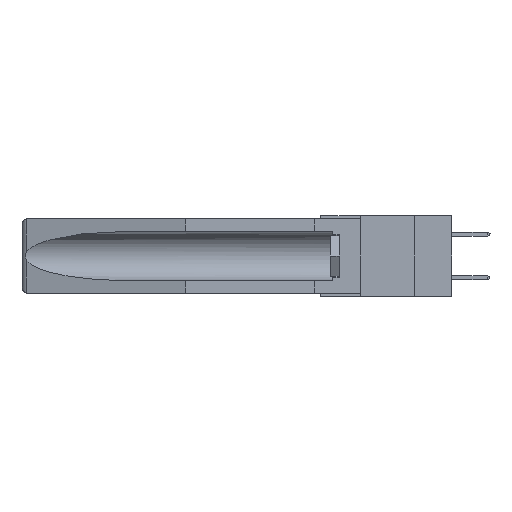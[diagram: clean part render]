
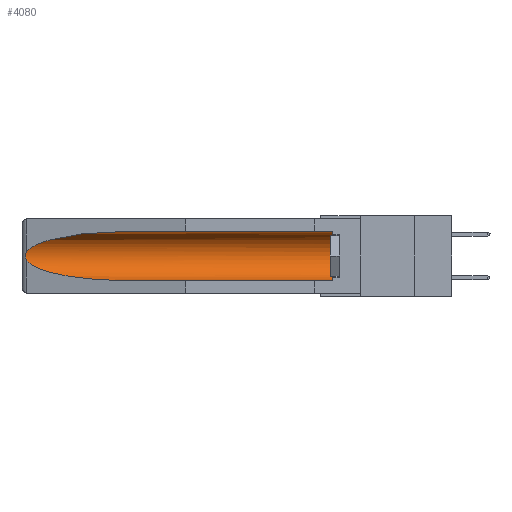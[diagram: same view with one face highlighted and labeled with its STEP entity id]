
A CAD part, left-side view. The second image highlights one B-rep face of the part: STEP entity #4080.
In plain terms, the highlighted cylindrical face has radius 2.857 mm (diameter 5.715 mm), a partial arc.
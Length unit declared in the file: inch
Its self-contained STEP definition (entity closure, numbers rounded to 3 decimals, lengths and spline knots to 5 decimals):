
#59 = LINE ( 'NONE', #6340, #12403 ) ;
#96 = ORIENTED_EDGE ( 'NONE', *, *, #6446, .F. ) ;
#229 = EDGE_CURVE ( 'NONE', #886, #3512, #5352, .T. ) ;
#364 = CARTESIAN_POINT ( 'NONE',  ( 0.26537, 1.52718, -0.14972 ) ) ;
#886 = VERTEX_POINT ( 'NONE', #3057 ) ;
#1136 = EDGE_CURVE ( 'NONE', #8082, #19232, #3600, .T. ) ;
#1971 = EDGE_CURVE ( 'NONE', #3512, #8082, #18504, .T. ) ;
#1979 = CYLINDRICAL_SURFACE ( 'NONE', #12974, 0.1125 ) ;
#2061 = CARTESIAN_POINT ( 'NONE',  ( 0.26655, 1.53094, -0.18657 ) ) ;
#2127 = CARTESIAN_POINT ( 'NONE',  ( 0.26597, 1.5296, -0.19026 ) ) ;
#3057 = CARTESIAN_POINT ( 'NONE',  ( 0.155, 1.07973, -0.059 ) ) ;
#3501 = VERTEX_POINT ( 'NONE', #14942 ) ;
#3512 = VERTEX_POINT ( 'NONE', #10009 ) ;
#3600 =( BOUNDED_CURVE ( )  B_SPLINE_CURVE ( 3, ( #16411, #5710, #16742, #4212 ),
 .UNSPECIFIED., .F., .F. ) 
 B_SPLINE_CURVE_WITH_KNOTS ( ( 4, 4 ),
 ( 0.1948, 1.5708 ),
 .UNSPECIFIED. ) 
 CURVE ( )  GEOMETRIC_REPRESENTATION_ITEM ( )  RATIONAL_B_SPLINE_CURVE ( ( 1., 0.848, 0.848, 1. ) ) 
 REPRESENTATION_ITEM ( '' )  );
#4080 = ADVANCED_FACE ( 'NONE', ( #11611 ), #1979, .F. ) ;
#4212 = CARTESIAN_POINT ( 'NONE',  ( 0.155, 1.07973, -0.284 ) ) ;
#4450 = ORIENTED_EDGE ( 'NONE', *, *, #1136, .T. ) ;
#4762 = CARTESIAN_POINT ( 'NONE',  ( 0.155, 0.126, -0.059 ) ) ;
#4929 = DIRECTION ( 'NONE',  ( 0., 0., 1. ) ) ;
#5352 =( BOUNDED_CURVE ( )  B_SPLINE_CURVE ( 3, ( #9157, #12213, #19887, #10605 ),
 .UNSPECIFIED., .F., .F. ) 
 B_SPLINE_CURVE_WITH_KNOTS ( ( 4, 4 ),
 ( 4.71239, 6.08839 ),
 .UNSPECIFIED. ) 
 CURVE ( )  GEOMETRIC_REPRESENTATION_ITEM ( )  RATIONAL_B_SPLINE_CURVE ( ( 1., 0.848, 0.848, 1. ) ) 
 REPRESENTATION_ITEM ( '' )  );
#5520 = VECTOR ( 'NONE', #10115, 39.37008 ) ;
#5608 = CARTESIAN_POINT ( 'NONE',  ( 0.155, -0.30754, -0.284 ) ) ;
#5710 = CARTESIAN_POINT ( 'NONE',  ( 0.25451, 1.48313, -0.24835 ) ) ;
#6310 = EDGE_LOOP ( 'NONE', ( #19015, #10047, #4450, #96, #11923, #17736 ) ) ;
#6340 = CARTESIAN_POINT ( 'NONE',  ( 0.155, -0.30754, -0.059 ) ) ;
#6446 = EDGE_CURVE ( 'NONE', #3501, #19232, #12207, .T. ) ;
#7437 = EDGE_CURVE ( 'NONE', #16050, #886, #59, .T. ) ;
#7913 = CARTESIAN_POINT ( 'NONE',  ( 0.2675, 1.53308, -0.17534 ) ) ;
#8082 = VERTEX_POINT ( 'NONE', #12690 ) ;
#8116 = DIRECTION ( 'NONE',  ( 0., 1., 0. ) ) ;
#9157 = CARTESIAN_POINT ( 'NONE',  ( 0.155, 1.07973, -0.059 ) ) ;
#9991 = CARTESIAN_POINT ( 'NONE',  ( 0.155, -0.30754, -0.1715 ) ) ;
#10009 = CARTESIAN_POINT ( 'NONE',  ( 0.26537, 1.52718, -0.14972 ) ) ;
#10047 = ORIENTED_EDGE ( 'NONE', *, *, #1971, .T. ) ;
#10115 = DIRECTION ( 'NONE',  ( 0., 1., 0. ) ) ;
#10605 = CARTESIAN_POINT ( 'NONE',  ( 0.26537, 1.52718, -0.14972 ) ) ;
#11555 = AXIS2_PLACEMENT_3D ( 'NONE', #16537, #18340, #19825 ) ;
#11611 = FACE_OUTER_BOUND ( 'NONE', #6310, .T. ) ;
#11923 = ORIENTED_EDGE ( 'NONE', *, *, #19619, .T. ) ;
#12207 = LINE ( 'NONE', #5608, #5520 ) ;
#12213 = CARTESIAN_POINT ( 'NONE',  ( 0.21114, 1.30732, -0.059 ) ) ;
#12403 = VECTOR ( 'NONE', #8116, 39.37008 ) ;
#12690 = CARTESIAN_POINT ( 'NONE',  ( 0.26537, 1.52718, -0.19328 ) ) ;
#12974 = AXIS2_PLACEMENT_3D ( 'NONE', #9991, #13154, #4929 ) ;
#12976 = CARTESIAN_POINT ( 'NONE',  ( 0.26597, 1.52961, -0.15275 ) ) ;
#13154 = DIRECTION ( 'NONE',  ( 0., 1., 0. ) ) ;
#14532 = CARTESIAN_POINT ( 'NONE',  ( 0.26654, 1.53092, -0.15636 ) ) ;
#14942 = CARTESIAN_POINT ( 'NONE',  ( 0.155, 0.126, -0.284 ) ) ;
#15355 = CIRCLE ( 'NONE', #11555, 0.1125 ) ;
#15520 = CARTESIAN_POINT ( 'NONE',  ( 0.155, 1.07973, -0.284 ) ) ;
#16050 = VERTEX_POINT ( 'NONE', #4762 ) ;
#16130 = CARTESIAN_POINT ( 'NONE',  ( 0.2673, 1.5327, -0.16383 ) ) ;
#16411 = CARTESIAN_POINT ( 'NONE',  ( 0.26537, 1.52718, -0.19328 ) ) ;
#16537 = CARTESIAN_POINT ( 'NONE',  ( 0.155, 0.126, -0.1715 ) ) ;
#16742 = CARTESIAN_POINT ( 'NONE',  ( 0.21114, 1.30732, -0.284 ) ) ;
#17381 = CARTESIAN_POINT ( 'NONE',  ( 0.2675, 1.53308, -0.16763 ) ) ;
#17736 = ORIENTED_EDGE ( 'NONE', *, *, #7437, .T. ) ;
#17914 = CARTESIAN_POINT ( 'NONE',  ( 0.26537, 1.52718, -0.19328 ) ) ;
#18340 = DIRECTION ( 'NONE',  ( 0., -1., 0. ) ) ;
#18504 = B_SPLINE_CURVE_WITH_KNOTS ( 'NONE', 3,
 ( #364, #12976, #14532, #16130, #17381, #7913, #19407, #2061, #2127, #17914 ),
 .UNSPECIFIED., .F., .F.,
 ( 4, 2, 2, 2, 4 ),
 ( 0., 0.00029, 0.00058, 0.00087, 0.00117 ),
 .UNSPECIFIED. ) ;
#19015 = ORIENTED_EDGE ( 'NONE', *, *, #229, .T. ) ;
#19232 = VERTEX_POINT ( 'NONE', #15520 ) ;
#19407 = CARTESIAN_POINT ( 'NONE',  ( 0.2673, 1.53269, -0.17917 ) ) ;
#19619 = EDGE_CURVE ( 'NONE', #3501, #16050, #15355, .T. ) ;
#19825 = DIRECTION ( 'NONE',  ( 0., 0., 1. ) ) ;
#19887 = CARTESIAN_POINT ( 'NONE',  ( 0.25451, 1.48313, -0.09465 ) ) ;
